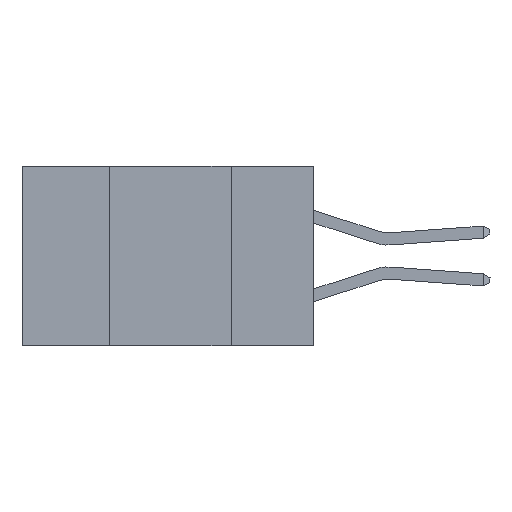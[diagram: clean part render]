
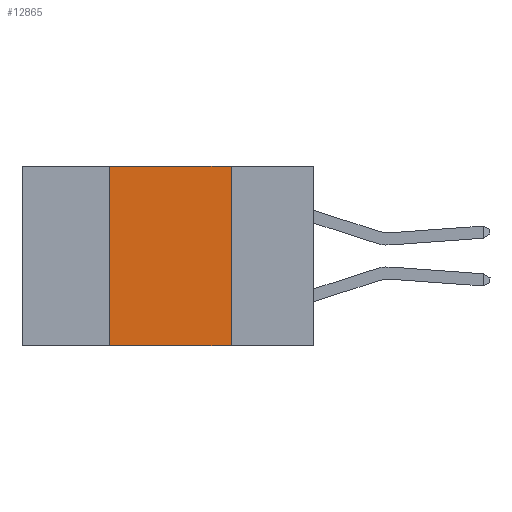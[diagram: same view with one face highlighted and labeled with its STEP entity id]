
A CAD part, left-side view. The second image highlights one B-rep face of the part: STEP entity #12865.
In plain terms, the highlighted planar face has unit normal (-1, 0, 0).
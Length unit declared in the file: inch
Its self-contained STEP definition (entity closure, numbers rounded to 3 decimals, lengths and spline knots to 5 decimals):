
#909 = VECTOR ( 'NONE', #3881, 39.37008 ) ;
#1607 = VERTEX_POINT ( 'NONE', #16201 ) ;
#1757 = EDGE_CURVE ( 'NONE', #6752, #16486, #4096, .T. ) ;
#2689 = EDGE_CURVE ( 'NONE', #6752, #1607, #8354, .T. ) ;
#2817 = AXIS2_PLACEMENT_3D ( 'NONE', #10217, #6055, #15894 ) ;
#3759 = FACE_OUTER_BOUND ( 'NONE', #8229, .T. ) ;
#3881 = DIRECTION ( 'NONE',  ( 0., -1., 0. ) ) ;
#4096 = LINE ( 'NONE', #14406, #11145 ) ;
#4927 = LINE ( 'NONE', #7088, #11990 ) ;
#5904 = CARTESIAN_POINT ( 'NONE',  ( 0., 0.6, 0. ) ) ;
#6055 = DIRECTION ( 'NONE',  ( 1., 0., 0. ) ) ;
#6203 = VECTOR ( 'NONE', #7317, 39.37008 ) ;
#6417 = EDGE_CURVE ( 'NONE', #6820, #1607, #4927, .T. ) ;
#6752 = VERTEX_POINT ( 'NONE', #13414 ) ;
#6820 = VERTEX_POINT ( 'NONE', #14972 ) ;
#7088 = CARTESIAN_POINT ( 'NONE',  ( 0., 0.17, 0. ) ) ;
#7215 = EDGE_CURVE ( 'NONE', #16486, #6820, #17413, .T. ) ;
#7317 = DIRECTION ( 'NONE',  ( 0., -1., 0. ) ) ;
#8229 = EDGE_LOOP ( 'NONE', ( #9499, #9546, #9613, #9646 ) ) ;
#8354 = LINE ( 'NONE', #9529, #909 ) ;
#8528 = DIRECTION ( 'NONE',  ( 0., 0., -1. ) ) ;
#8831 = PLANE ( 'NONE',  #2817 ) ;
#9499 = ORIENTED_EDGE ( 'NONE', *, *, #6417, .F. ) ;
#9529 = CARTESIAN_POINT ( 'NONE',  ( 0., 0.6, -0.37 ) ) ;
#9546 = ORIENTED_EDGE ( 'NONE', *, *, #7215, .F. ) ;
#9613 = ORIENTED_EDGE ( 'NONE', *, *, #1757, .F. ) ;
#9646 = ORIENTED_EDGE ( 'NONE', *, *, #2689, .T. ) ;
#10217 = CARTESIAN_POINT ( 'NONE',  ( 0., 0.6, 0. ) ) ;
#11145 = VECTOR ( 'NONE', #15813, 39.37008 ) ;
#11990 = VECTOR ( 'NONE', #8528, 39.37008 ) ;
#12865 = ADVANCED_FACE ( 'NONE', ( #3759 ), #8831, .F. ) ;
#13414 = CARTESIAN_POINT ( 'NONE',  ( 0., 0.42, -0.37 ) ) ;
#14277 = CARTESIAN_POINT ( 'NONE',  ( 0., 0.42, 0. ) ) ;
#14406 = CARTESIAN_POINT ( 'NONE',  ( 0., 0.42, 0. ) ) ;
#14972 = CARTESIAN_POINT ( 'NONE',  ( 0., 0.17, 0. ) ) ;
#15813 = DIRECTION ( 'NONE',  ( 0., 0., 1. ) ) ;
#15894 = DIRECTION ( 'NONE',  ( 0., 0., -1. ) ) ;
#16201 = CARTESIAN_POINT ( 'NONE',  ( 0., 0.17, -0.37 ) ) ;
#16486 = VERTEX_POINT ( 'NONE', #14277 ) ;
#17413 = LINE ( 'NONE', #5904, #6203 ) ;
